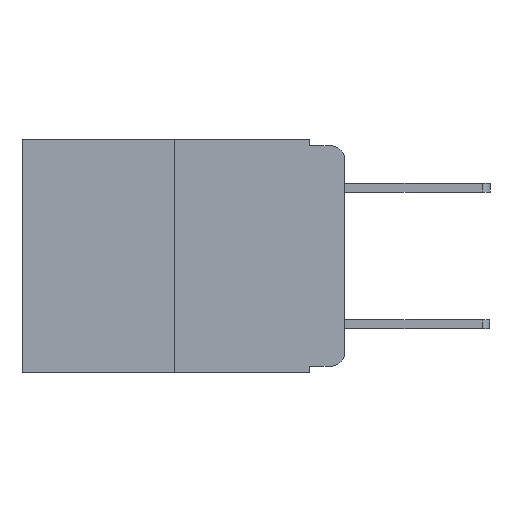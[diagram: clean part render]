
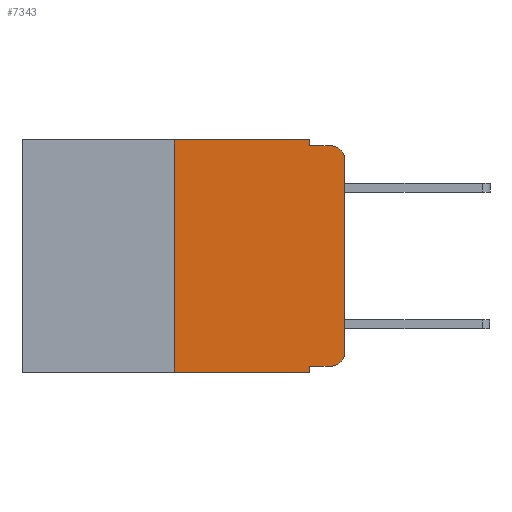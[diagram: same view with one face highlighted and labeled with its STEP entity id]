
A CAD part, left-side view. The second image highlights one B-rep face of the part: STEP entity #7343.
In plain terms, the highlighted planar face has unit normal (-1, 0, 0).
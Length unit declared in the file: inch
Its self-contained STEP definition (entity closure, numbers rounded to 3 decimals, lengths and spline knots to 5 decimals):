
#169 = ORIENTED_EDGE ( 'NONE', *, *, #7623, .T. ) ;
#212 = VECTOR ( 'NONE', #11673, 39.37008 ) ;
#652 = EDGE_CURVE ( 'NONE', #7673, #11639, #6037, .T. ) ;
#855 = CARTESIAN_POINT ( 'NONE',  ( 0., 0.02, -0.01 ) ) ;
#1936 = VERTEX_POINT ( 'NONE', #4472 ) ;
#2111 = VERTEX_POINT ( 'NONE', #8883 ) ;
#2115 = ORIENTED_EDGE ( 'NONE', *, *, #7030, .T. ) ;
#2312 = PLANE ( 'NONE',  #2991 ) ;
#2329 = CARTESIAN_POINT ( 'NONE',  ( 0., 0.051, -0.01 ) ) ;
#2410 = CARTESIAN_POINT ( 'NONE',  ( 0., 0.051, 0. ) ) ;
#2696 = CARTESIAN_POINT ( 'NONE',  ( 0., 0.051, -0.01 ) ) ;
#2772 = CARTESIAN_POINT ( 'NONE',  ( 0., 0.473, -0.343 ) ) ;
#2991 = AXIS2_PLACEMENT_3D ( 'NONE', #3410, #4474, #10925 ) ;
#3410 = CARTESIAN_POINT ( 'NONE',  ( 0., 0.473, 0. ) ) ;
#3473 = VERTEX_POINT ( 'NONE', #11268 ) ;
#3495 = DIRECTION ( 'NONE',  ( 0., 0., -1. ) ) ;
#3562 = CARTESIAN_POINT ( 'NONE',  ( 0., 0.051, 0. ) ) ;
#4099 = VECTOR ( 'NONE', #3495, 39.37008 ) ;
#4326 = CARTESIAN_POINT ( 'NONE',  ( 0., 0.051, -0.333 ) ) ;
#4364 = CARTESIAN_POINT ( 'NONE',  ( 0., 0.051, 0. ) ) ;
#4456 = DIRECTION ( 'NONE',  ( -1., 0., 0. ) ) ;
#4472 = CARTESIAN_POINT ( 'NONE',  ( 0., 0.051, -0.343 ) ) ;
#4474 = DIRECTION ( 'NONE',  ( 1., 0., 0. ) ) ;
#4765 = LINE ( 'NONE', #8167, #9540 ) ;
#4770 = VERTEX_POINT ( 'NONE', #7978 ) ;
#4814 = LINE ( 'NONE', #4364, #11947 ) ;
#4833 = VERTEX_POINT ( 'NONE', #4326 ) ;
#5333 = ORIENTED_EDGE ( 'NONE', *, *, #7361, .F. ) ;
#6037 = LINE ( 'NONE', #7478, #212 ) ;
#6249 = EDGE_CURVE ( 'NONE', #2111, #3473, #6941, .T. ) ;
#6265 = DIRECTION ( 'NONE',  ( -1., 0., 0. ) ) ;
#6297 = DIRECTION ( 'NONE',  ( 0., -1., 0. ) ) ;
#6299 = LINE ( 'NONE', #8234, #10446 ) ;
#6377 = EDGE_CURVE ( 'NONE', #3473, #10249, #11334, .T. ) ;
#6630 = EDGE_CURVE ( 'NONE', #8197, #10249, #6779, .T. ) ;
#6779 = LINE ( 'NONE', #2696, #8942 ) ;
#6834 = EDGE_CURVE ( 'NONE', #11639, #8197, #4814, .T. ) ;
#6941 = LINE ( 'NONE', #11365, #11225 ) ;
#7030 = EDGE_CURVE ( 'NONE', #4770, #1936, #8367, .T. ) ;
#7170 = EDGE_CURVE ( 'NONE', #4770, #7673, #6299, .T. ) ;
#7343 = ADVANCED_FACE ( 'NONE', ( #7484 ), #2312, .F. ) ;
#7361 = EDGE_CURVE ( 'NONE', #4833, #1936, #11414, .T. ) ;
#7368 = ORIENTED_EDGE ( 'NONE', *, *, #7170, .F. ) ;
#7478 = CARTESIAN_POINT ( 'NONE',  ( 0., 0.473, 0. ) ) ;
#7484 = FACE_OUTER_BOUND ( 'NONE', #11253, .T. ) ;
#7616 = CIRCLE ( 'NONE', #10980, 0.02 ) ;
#7623 = EDGE_CURVE ( 'NONE', #4833, #9616, #4765, .T. ) ;
#7630 = ORIENTED_EDGE ( 'NONE', *, *, #652, .F. ) ;
#7673 = VERTEX_POINT ( 'NONE', #9938 ) ;
#7772 = EDGE_CURVE ( 'NONE', #9616, #2111, #7616, .T. ) ;
#7781 = ORIENTED_EDGE ( 'NONE', *, *, #6377, .T. ) ;
#7925 = ORIENTED_EDGE ( 'NONE', *, *, #6249, .T. ) ;
#7978 = CARTESIAN_POINT ( 'NONE',  ( 0., 0.25, -0.343 ) ) ;
#8077 = ORIENTED_EDGE ( 'NONE', *, *, #6630, .F. ) ;
#8167 = CARTESIAN_POINT ( 'NONE',  ( 0., 0.051, -0.333 ) ) ;
#8197 = VERTEX_POINT ( 'NONE', #2329 ) ;
#8234 = CARTESIAN_POINT ( 'NONE',  ( 0., 0.25, 0. ) ) ;
#8367 = LINE ( 'NONE', #2772, #8919 ) ;
#8883 = CARTESIAN_POINT ( 'NONE',  ( 0., 0., -0.313 ) ) ;
#8919 = VECTOR ( 'NONE', #11216, 39.37008 ) ;
#8942 = VECTOR ( 'NONE', #11962, 39.37008 ) ;
#9540 = VECTOR ( 'NONE', #6297, 39.37008 ) ;
#9616 = VERTEX_POINT ( 'NONE', #11151 ) ;
#9692 = AXIS2_PLACEMENT_3D ( 'NONE', #11435, #6265, #12223 ) ;
#9938 = CARTESIAN_POINT ( 'NONE',  ( 0., 0.25, 0. ) ) ;
#10107 = CARTESIAN_POINT ( 'NONE',  ( 0., 0.02, -0.313 ) ) ;
#10249 = VERTEX_POINT ( 'NONE', #855 ) ;
#10446 = VECTOR ( 'NONE', #12272, 39.37008 ) ;
#10710 = ORIENTED_EDGE ( 'NONE', *, *, #7772, .T. ) ;
#10842 = DIRECTION ( 'NONE',  ( 0., 0., -1. ) ) ;
#10909 = DIRECTION ( 'NONE',  ( 0., 0., -1. ) ) ;
#10925 = DIRECTION ( 'NONE',  ( 0., 0., -1. ) ) ;
#10980 = AXIS2_PLACEMENT_3D ( 'NONE', #10107, #4456, #10909 ) ;
#11151 = CARTESIAN_POINT ( 'NONE',  ( 0., 0.02, -0.333 ) ) ;
#11216 = DIRECTION ( 'NONE',  ( 0., -1., 0. ) ) ;
#11225 = VECTOR ( 'NONE', #12169, 39.37008 ) ;
#11253 = EDGE_LOOP ( 'NONE', ( #7925, #7781, #8077, #11295, #7630, #7368, #2115, #5333, #169, #10710 ) ) ;
#11268 = CARTESIAN_POINT ( 'NONE',  ( 0., 0., -0.03 ) ) ;
#11295 = ORIENTED_EDGE ( 'NONE', *, *, #6834, .F. ) ;
#11334 = CIRCLE ( 'NONE', #9692, 0.02 ) ;
#11365 = CARTESIAN_POINT ( 'NONE',  ( 0., 0., 0. ) ) ;
#11414 = LINE ( 'NONE', #2410, #4099 ) ;
#11435 = CARTESIAN_POINT ( 'NONE',  ( 0., 0.02, -0.03 ) ) ;
#11639 = VERTEX_POINT ( 'NONE', #3562 ) ;
#11673 = DIRECTION ( 'NONE',  ( 0., -1., 0. ) ) ;
#11947 = VECTOR ( 'NONE', #10842, 39.37008 ) ;
#11962 = DIRECTION ( 'NONE',  ( 0., -1., 0. ) ) ;
#12169 = DIRECTION ( 'NONE',  ( 0., 0., 1. ) ) ;
#12223 = DIRECTION ( 'NONE',  ( 0., 0., -1. ) ) ;
#12272 = DIRECTION ( 'NONE',  ( 0., 0., 1. ) ) ;
